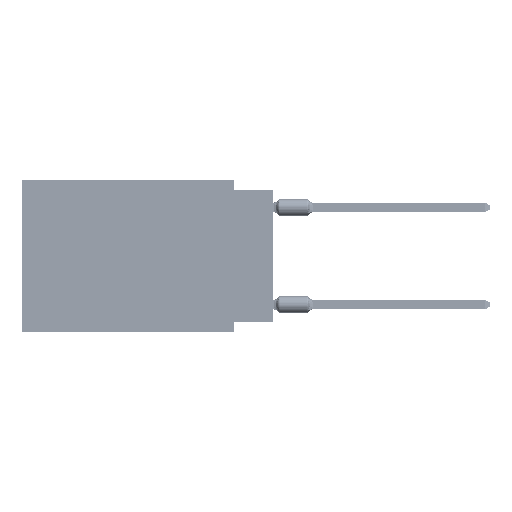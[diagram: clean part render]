
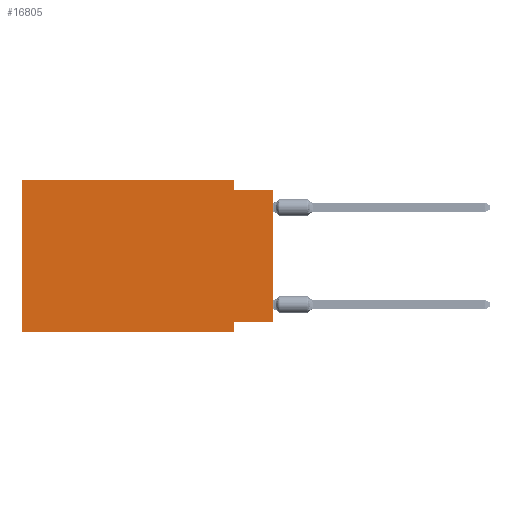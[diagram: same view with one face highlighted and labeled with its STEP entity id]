
A CAD part, left-side view. The second image highlights one B-rep face of the part: STEP entity #16805.
In plain terms, the highlighted planar face has unit normal (-1, 0, 0).
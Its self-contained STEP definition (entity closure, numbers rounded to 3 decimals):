
#653 = FACE_OUTER_BOUND ( 'NONE', #5594, .T. ) ;
#1001 = DIRECTION ( 'NONE',  ( 0., 0., -1. ) ) ;
#2455 = VERTEX_POINT ( 'NONE', #6159 ) ;
#2628 = ORIENTED_EDGE ( 'NONE', *, *, #12600, .F. ) ;
#4497 = CARTESIAN_POINT ( 'NONE',  ( 0., 0., -9.271 ) ) ;
#4585 = VECTOR ( 'NONE', #17715, 1000. ) ;
#5034 = LINE ( 'NONE', #16533, #49342 ) ;
#5594 = EDGE_LOOP ( 'NONE', ( #48701, #2628, #13274, #36645, #46681, #6006, #64900, #27065 ) ) ;
#5804 = CARTESIAN_POINT ( 'NONE',  ( 0., 16.383, 0. ) ) ;
#5982 = VECTOR ( 'NONE', #24144, 1000. ) ;
#6006 = ORIENTED_EDGE ( 'NONE', *, *, #69019, .T. ) ;
#6057 = DIRECTION ( 'NONE',  ( 0., -1., 0. ) ) ;
#6159 = CARTESIAN_POINT ( 'NONE',  ( 0., 2.54, -9.271 ) ) ;
#9374 = DIRECTION ( 'NONE',  ( 0., 1., 0. ) ) ;
#12591 = VECTOR ( 'NONE', #9374, 1000. ) ;
#12600 = EDGE_CURVE ( 'NONE', #60450, #21606, #35923, .T. ) ;
#13274 = ORIENTED_EDGE ( 'NONE', *, *, #49484, .F. ) ;
#13748 = CARTESIAN_POINT ( 'NONE',  ( 0., 0., -9.271 ) ) ;
#14683 = VECTOR ( 'NONE', #64009, 1000. ) ;
#16533 = CARTESIAN_POINT ( 'NONE',  ( 0., 16.383, 0. ) ) ;
#16690 = PLANE ( 'NONE',  #55515 ) ;
#16805 = ADVANCED_FACE ( 'NONE', ( #653 ), #16690, .F. ) ;
#17715 = DIRECTION ( 'NONE',  ( 0., 0., -1. ) ) ;
#18850 = EDGE_CURVE ( 'NONE', #26427, #19816, #5034, .T. ) ;
#19816 = VERTEX_POINT ( 'NONE', #50160 ) ;
#20366 = CARTESIAN_POINT ( 'NONE',  ( 0., 16.383, 0. ) ) ;
#21606 = VERTEX_POINT ( 'NONE', #37483 ) ;
#23319 = EDGE_CURVE ( 'NONE', #64865, #2455, #56173, .T. ) ;
#24144 = DIRECTION ( 'NONE',  ( 0., 0., 1. ) ) ;
#24184 = DIRECTION ( 'NONE',  ( 0., 0., -1. ) ) ;
#24388 = LINE ( 'NONE', #56154, #31792 ) ;
#25079 = DIRECTION ( 'NONE',  ( 0., -1., 0. ) ) ;
#26427 = VERTEX_POINT ( 'NONE', #5804 ) ;
#27065 = ORIENTED_EDGE ( 'NONE', *, *, #23319, .F. ) ;
#28951 = EDGE_CURVE ( 'NONE', #2455, #59118, #34661, .T. ) ;
#30360 = CARTESIAN_POINT ( 'NONE',  ( 0., 0., -0.635 ) ) ;
#30706 = DIRECTION ( 'NONE',  ( 0., -1., 0. ) ) ;
#31792 = VECTOR ( 'NONE', #25079, 1000. ) ;
#34170 = EDGE_CURVE ( 'NONE', #38385, #26427, #52496, .T. ) ;
#34279 = LINE ( 'NONE', #44754, #5982 ) ;
#34661 = LINE ( 'NONE', #55957, #60115 ) ;
#35923 = LINE ( 'NONE', #30360, #50844 ) ;
#36645 = ORIENTED_EDGE ( 'NONE', *, *, #18850, .F. ) ;
#37483 = CARTESIAN_POINT ( 'NONE',  ( 0., 0., -0.635 ) ) ;
#38385 = VERTEX_POINT ( 'NONE', #68986 ) ;
#44754 = CARTESIAN_POINT ( 'NONE',  ( 0., 0., 0. ) ) ;
#46681 = ORIENTED_EDGE ( 'NONE', *, *, #34170, .F. ) ;
#47786 = CARTESIAN_POINT ( 'NONE',  ( 0., 16.383, 0. ) ) ;
#48701 = ORIENTED_EDGE ( 'NONE', *, *, #65303, .T. ) ;
#49342 = VECTOR ( 'NONE', #6057, 1000. ) ;
#49484 = EDGE_CURVE ( 'NONE', #19816, #60450, #59971, .T. ) ;
#50160 = CARTESIAN_POINT ( 'NONE',  ( 0., 2.54, 0. ) ) ;
#50844 = VECTOR ( 'NONE', #30706, 1000. ) ;
#52496 = LINE ( 'NONE', #20366, #14683 ) ;
#55515 = AXIS2_PLACEMENT_3D ( 'NONE', #47786, #64552, #1001 ) ;
#55957 = CARTESIAN_POINT ( 'NONE',  ( 0., 2.54, -9.906 ) ) ;
#56154 = CARTESIAN_POINT ( 'NONE',  ( 0., 16.383, -9.906 ) ) ;
#56173 = LINE ( 'NONE', #4497, #12591 ) ;
#56613 = CARTESIAN_POINT ( 'NONE',  ( 0., 2.54, -0.635 ) ) ;
#59118 = VERTEX_POINT ( 'NONE', #65386 ) ;
#59971 = LINE ( 'NONE', #65568, #4585 ) ;
#60115 = VECTOR ( 'NONE', #24184, 1000. ) ;
#60450 = VERTEX_POINT ( 'NONE', #56613 ) ;
#64009 = DIRECTION ( 'NONE',  ( 0., 0., 1. ) ) ;
#64552 = DIRECTION ( 'NONE',  ( 1., 0., 0. ) ) ;
#64865 = VERTEX_POINT ( 'NONE', #13748 ) ;
#64900 = ORIENTED_EDGE ( 'NONE', *, *, #28951, .F. ) ;
#65303 = EDGE_CURVE ( 'NONE', #64865, #21606, #34279, .T. ) ;
#65386 = CARTESIAN_POINT ( 'NONE',  ( 0., 2.54, -9.906 ) ) ;
#65568 = CARTESIAN_POINT ( 'NONE',  ( 0., 2.54, 0. ) ) ;
#68986 = CARTESIAN_POINT ( 'NONE',  ( 0., 16.383, -9.906 ) ) ;
#69019 = EDGE_CURVE ( 'NONE', #38385, #59118, #24388, .T. ) ;
